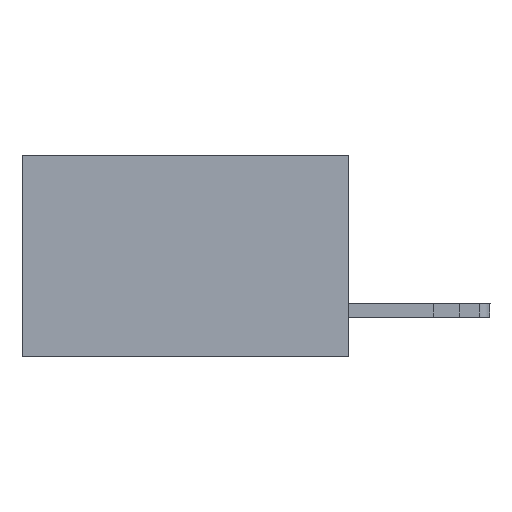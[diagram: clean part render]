
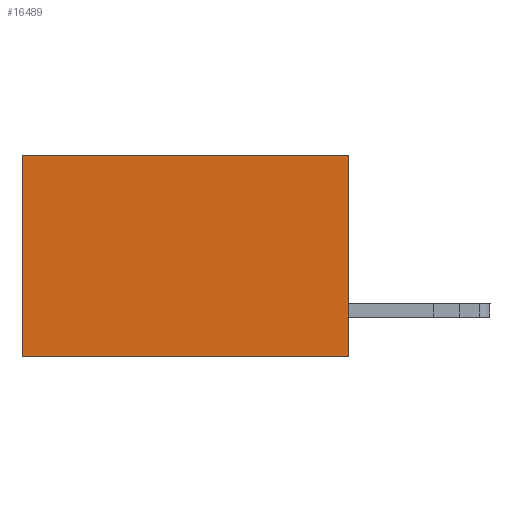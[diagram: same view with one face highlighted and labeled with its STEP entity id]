
A CAD part, left-side view. The second image highlights one B-rep face of the part: STEP entity #16489.
In plain terms, the highlighted planar face has unit normal (-1, 0, 0).
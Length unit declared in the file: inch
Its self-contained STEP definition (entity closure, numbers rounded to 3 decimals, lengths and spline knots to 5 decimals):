
#33 = DIRECTION ( 'NONE',  ( 0., 0., -1. ) ) ;
#290 = CARTESIAN_POINT ( 'NONE',  ( 0.2615, 0., -0.37 ) ) ;
#641 = CARTESIAN_POINT ( 'NONE',  ( 0.2615, 0., 0. ) ) ;
#1062 = EDGE_LOOP ( 'NONE', ( #6558, #15351, #8002, #5235 ) ) ;
#1809 = DIRECTION ( 'NONE',  ( 0., 1., 0. ) ) ;
#1876 = EDGE_CURVE ( 'NONE', #14213, #7665, #7117, .T. ) ;
#4538 = LINE ( 'NONE', #8691, #8945 ) ;
#5134 = EDGE_CURVE ( 'NONE', #15412, #15777, #11685, .T. ) ;
#5231 = CARTESIAN_POINT ( 'NONE',  ( 0.2615, 0., -0.37 ) ) ;
#5235 = ORIENTED_EDGE ( 'NONE', *, *, #5134, .T. ) ;
#5416 = DIRECTION ( 'NONE',  ( 0., 1., 0. ) ) ;
#6517 = FACE_OUTER_BOUND ( 'NONE', #1062, .T. ) ;
#6558 = ORIENTED_EDGE ( 'NONE', *, *, #16160, .T. ) ;
#7117 = LINE ( 'NONE', #15762, #18435 ) ;
#7532 = DIRECTION ( 'NONE',  ( 0., 0., -1. ) ) ;
#7665 = VERTEX_POINT ( 'NONE', #8399 ) ;
#8002 = ORIENTED_EDGE ( 'NONE', *, *, #17563, .F. ) ;
#8399 = CARTESIAN_POINT ( 'NONE',  ( 0.2615, 0.6, -0.37 ) ) ;
#8691 = CARTESIAN_POINT ( 'NONE',  ( 0.2615, 0.6, -0.37 ) ) ;
#8945 = VECTOR ( 'NONE', #33, 39.37008 ) ;
#9294 = VECTOR ( 'NONE', #7532, 39.37008 ) ;
#9988 = CARTESIAN_POINT ( 'NONE',  ( 0.2615, 0., 0. ) ) ;
#10086 = LINE ( 'NONE', #290, #9294 ) ;
#10966 = VECTOR ( 'NONE', #1809, 39.37008 ) ;
#11383 = DIRECTION ( 'NONE',  ( 0., 0., -1. ) ) ;
#11685 = LINE ( 'NONE', #9988, #10966 ) ;
#14059 = AXIS2_PLACEMENT_3D ( 'NONE', #16671, #16576, #11383 ) ;
#14201 = PLANE ( 'NONE',  #14059 ) ;
#14213 = VERTEX_POINT ( 'NONE', #5231 ) ;
#14553 = CARTESIAN_POINT ( 'NONE',  ( 0.2615, 0.6, 0. ) ) ;
#15351 = ORIENTED_EDGE ( 'NONE', *, *, #1876, .F. ) ;
#15412 = VERTEX_POINT ( 'NONE', #641 ) ;
#15762 = CARTESIAN_POINT ( 'NONE',  ( 0.2615, 0., -0.37 ) ) ;
#15777 = VERTEX_POINT ( 'NONE', #14553 ) ;
#16160 = EDGE_CURVE ( 'NONE', #15777, #7665, #4538, .T. ) ;
#16489 = ADVANCED_FACE ( 'NONE', ( #6517 ), #14201, .F. ) ;
#16576 = DIRECTION ( 'NONE',  ( 1., 0., 0. ) ) ;
#16671 = CARTESIAN_POINT ( 'NONE',  ( 0.2615, 0., -0.37 ) ) ;
#17563 = EDGE_CURVE ( 'NONE', #15412, #14213, #10086, .T. ) ;
#18435 = VECTOR ( 'NONE', #5416, 39.37008 ) ;
